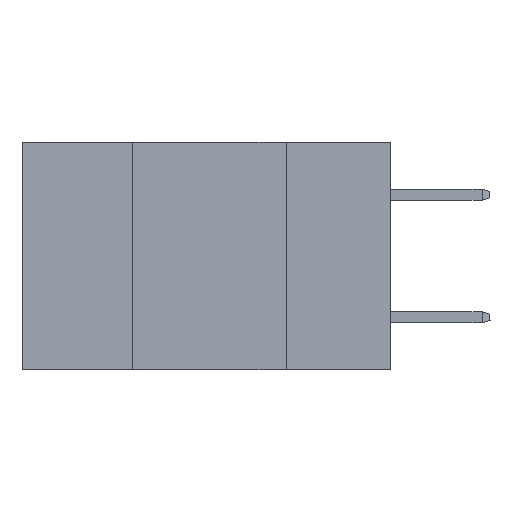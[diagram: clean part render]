
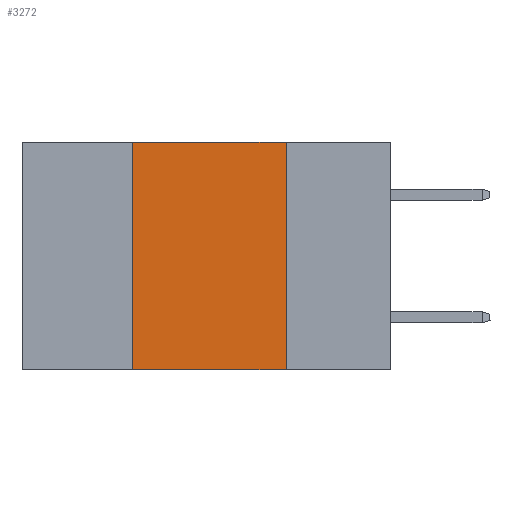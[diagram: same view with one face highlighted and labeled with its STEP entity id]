
A CAD part, left-side view. The second image highlights one B-rep face of the part: STEP entity #3272.
In plain terms, the highlighted planar face has unit normal (-1, 0, 0).
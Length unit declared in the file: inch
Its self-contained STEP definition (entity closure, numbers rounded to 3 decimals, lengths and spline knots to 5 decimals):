
#885 = AXIS2_PLACEMENT_3D ( 'NONE', #1850, #16246, #24336 ) ;
#1850 = CARTESIAN_POINT ( 'NONE',  ( 0., 0.6, 0. ) ) ;
#2408 = CARTESIAN_POINT ( 'NONE',  ( 0., 0.42, -0.37 ) ) ;
#3272 = ADVANCED_FACE ( 'NONE', ( #13027 ), #7970, .F. ) ;
#4556 = VERTEX_POINT ( 'NONE', #16266 ) ;
#5901 = VECTOR ( 'NONE', #11274, 39.37008 ) ;
#7677 = VECTOR ( 'NONE', #16434, 39.37008 ) ;
#7970 = PLANE ( 'NONE',  #885 ) ;
#8781 = EDGE_CURVE ( 'NONE', #12026, #4556, #12128, .T. ) ;
#9126 = EDGE_CURVE ( 'NONE', #13670, #4556, #23744, .T. ) ;
#9530 = DIRECTION ( 'NONE',  ( 0., -1., 0. ) ) ;
#10851 = VERTEX_POINT ( 'NONE', #25900 ) ;
#11245 = EDGE_CURVE ( 'NONE', #13670, #10851, #22918, .T. ) ;
#11274 = DIRECTION ( 'NONE',  ( 0., 0., 1. ) ) ;
#11630 = CARTESIAN_POINT ( 'NONE',  ( 0., 0.42, 0. ) ) ;
#12026 = VERTEX_POINT ( 'NONE', #13925 ) ;
#12128 = LINE ( 'NONE', #22430, #7677 ) ;
#13027 = FACE_OUTER_BOUND ( 'NONE', #19460, .T. ) ;
#13310 = VECTOR ( 'NONE', #9530, 39.37008 ) ;
#13670 = VERTEX_POINT ( 'NONE', #2408 ) ;
#13925 = CARTESIAN_POINT ( 'NONE',  ( 0., 0.17, 0. ) ) ;
#14023 = DIRECTION ( 'NONE',  ( 0., -1., 0. ) ) ;
#14991 = EDGE_CURVE ( 'NONE', #10851, #12026, #17196, .T. ) ;
#15418 = ORIENTED_EDGE ( 'NONE', *, *, #14991, .F. ) ;
#16246 = DIRECTION ( 'NONE',  ( 1., 0., 0. ) ) ;
#16266 = CARTESIAN_POINT ( 'NONE',  ( 0., 0.17, -0.37 ) ) ;
#16434 = DIRECTION ( 'NONE',  ( 0., 0., -1. ) ) ;
#16535 = ORIENTED_EDGE ( 'NONE', *, *, #9126, .T. ) ;
#17196 = LINE ( 'NONE', #21746, #13310 ) ;
#18322 = CARTESIAN_POINT ( 'NONE',  ( 0., 0.6, -0.37 ) ) ;
#19460 = EDGE_LOOP ( 'NONE', ( #21620, #15418, #26627, #16535 ) ) ;
#21620 = ORIENTED_EDGE ( 'NONE', *, *, #8781, .F. ) ;
#21746 = CARTESIAN_POINT ( 'NONE',  ( 0., 0.6, 0. ) ) ;
#22430 = CARTESIAN_POINT ( 'NONE',  ( 0., 0.17, 0. ) ) ;
#22918 = LINE ( 'NONE', #11630, #5901 ) ;
#23744 = LINE ( 'NONE', #18322, #26301 ) ;
#24336 = DIRECTION ( 'NONE',  ( 0., 0., -1. ) ) ;
#25900 = CARTESIAN_POINT ( 'NONE',  ( 0., 0.42, 0. ) ) ;
#26301 = VECTOR ( 'NONE', #14023, 39.37008 ) ;
#26627 = ORIENTED_EDGE ( 'NONE', *, *, #11245, .F. ) ;
